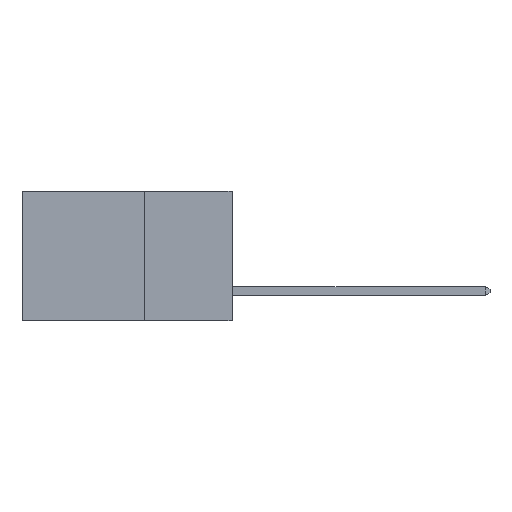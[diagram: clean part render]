
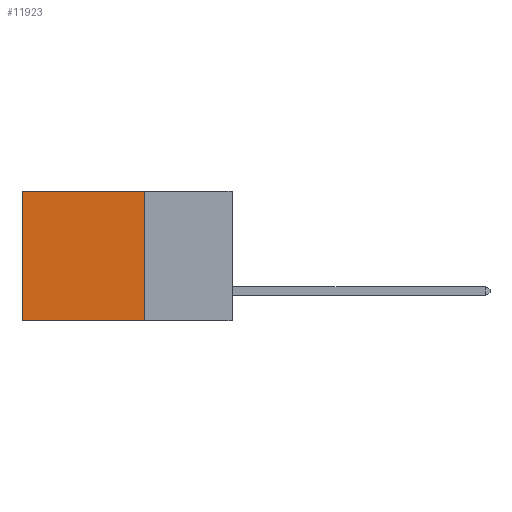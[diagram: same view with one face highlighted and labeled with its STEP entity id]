
A CAD part, left-side view. The second image highlights one B-rep face of the part: STEP entity #11923.
In plain terms, the highlighted planar face has unit normal (-1, 0, 0).
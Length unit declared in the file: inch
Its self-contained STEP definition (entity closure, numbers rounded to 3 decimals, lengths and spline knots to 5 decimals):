
#4 = DIRECTION ( 'NONE',  ( 0., 0., -1. ) ) ;
#362 = CARTESIAN_POINT ( 'NONE',  ( 0.2875, 0.25, -0.37 ) ) ;
#764 = CARTESIAN_POINT ( 'NONE',  ( 0.2875, 0.6, -0.37 ) ) ;
#1097 = VERTEX_POINT ( 'NONE', #23211 ) ;
#1752 = PLANE ( 'NONE',  #28252 ) ;
#2038 = ORIENTED_EDGE ( 'NONE', *, *, #17535, .T. ) ;
#4028 = ORIENTED_EDGE ( 'NONE', *, *, #26322, .F. ) ;
#4410 = LINE ( 'NONE', #13776, #18031 ) ;
#6503 = EDGE_CURVE ( 'NONE', #29631, #1097, #9715, .T. ) ;
#9501 = VERTEX_POINT ( 'NONE', #362 ) ;
#9715 = LINE ( 'NONE', #18307, #15260 ) ;
#11716 = ORIENTED_EDGE ( 'NONE', *, *, #22730, .F. ) ;
#11923 = ADVANCED_FACE ( 'NONE', ( #29544 ), #1752, .F. ) ;
#12784 = CARTESIAN_POINT ( 'NONE',  ( 0.2875, 0.25, 0. ) ) ;
#13776 = CARTESIAN_POINT ( 'NONE',  ( 0.2875, 0.25, 0. ) ) ;
#15260 = VECTOR ( 'NONE', #33807, 39.37008 ) ;
#15567 = DIRECTION ( 'NONE',  ( 1., 0., 0. ) ) ;
#16449 = ORIENTED_EDGE ( 'NONE', *, *, #6503, .T. ) ;
#17195 = EDGE_LOOP ( 'NONE', ( #2038, #4028, #11716, #16449 ) ) ;
#17205 = DIRECTION ( 'NONE',  ( 0., 1., 0. ) ) ;
#17223 = CARTESIAN_POINT ( 'NONE',  ( 0.2875, 0.6, 0. ) ) ;
#17535 = EDGE_CURVE ( 'NONE', #1097, #33234, #20171, .T. ) ;
#18031 = VECTOR ( 'NONE', #4, 39.37008 ) ;
#18307 = CARTESIAN_POINT ( 'NONE',  ( 0.2875, 0.25, 0. ) ) ;
#18564 = VECTOR ( 'NONE', #22492, 39.37008 ) ;
#20171 = LINE ( 'NONE', #17223, #18564 ) ;
#22095 = VECTOR ( 'NONE', #17205, 39.37008 ) ;
#22492 = DIRECTION ( 'NONE',  ( 0., 0., -1. ) ) ;
#22730 = EDGE_CURVE ( 'NONE', #29631, #9501, #4410, .T. ) ;
#23211 = CARTESIAN_POINT ( 'NONE',  ( 0.2875, 0.6, 0. ) ) ;
#25316 = LINE ( 'NONE', #30157, #22095 ) ;
#26322 = EDGE_CURVE ( 'NONE', #9501, #33234, #25316, .T. ) ;
#28252 = AXIS2_PLACEMENT_3D ( 'NONE', #12784, #15567, #33755 ) ;
#29544 = FACE_OUTER_BOUND ( 'NONE', #17195, .T. ) ;
#29631 = VERTEX_POINT ( 'NONE', #30545 ) ;
#30157 = CARTESIAN_POINT ( 'NONE',  ( 0.2875, 0.25, -0.37 ) ) ;
#30545 = CARTESIAN_POINT ( 'NONE',  ( 0.2875, 0.25, 0. ) ) ;
#33234 = VERTEX_POINT ( 'NONE', #764 ) ;
#33755 = DIRECTION ( 'NONE',  ( 0., 0., -1. ) ) ;
#33807 = DIRECTION ( 'NONE',  ( 0., 1., 0. ) ) ;
